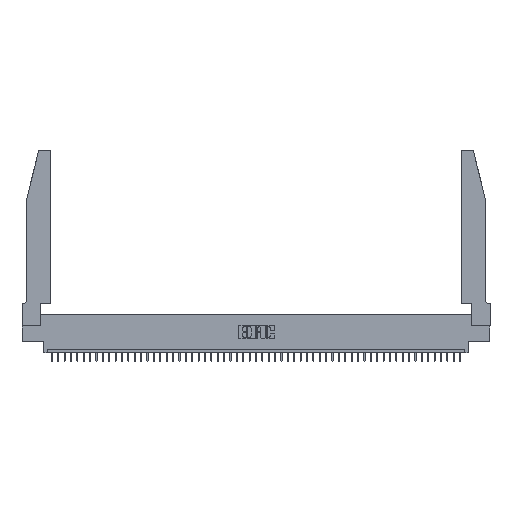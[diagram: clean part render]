
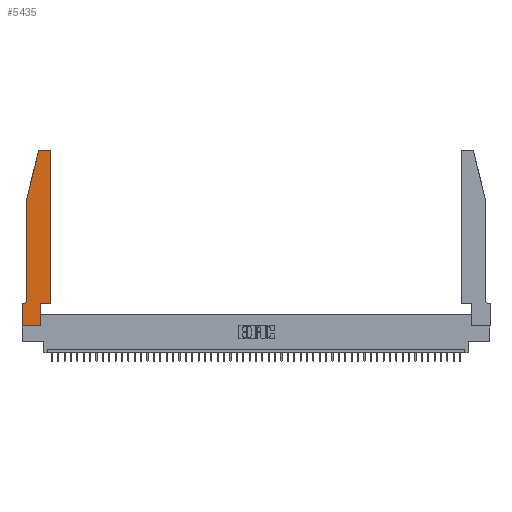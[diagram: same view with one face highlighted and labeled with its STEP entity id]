
A CAD part, top view. The second image highlights one B-rep face of the part: STEP entity #5435.
In plain terms, the highlighted planar face has unit normal (0, 0, 1).
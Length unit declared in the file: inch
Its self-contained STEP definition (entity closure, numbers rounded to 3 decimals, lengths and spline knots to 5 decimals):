
#126 = EDGE_CURVE ( 'NONE', #18314, #700, #9618, .T. ) ;
#479 = LINE ( 'NONE', #7968, #13682 ) ;
#640 = AXIS2_PLACEMENT_3D ( 'NONE', #26061, #41718, #37864 ) ;
#659 = LINE ( 'NONE', #17778, #2431 ) ;
#700 = VERTEX_POINT ( 'NONE', #10744 ) ;
#763 = EDGE_LOOP ( 'NONE', ( #3372, #18200, #48380, #49250, #43795, #35505, #13718, #44200, #23220, #9149, #31570, #44860 ) ) ;
#1346 = DIRECTION ( 'NONE',  ( -1., 0., 0. ) ) ;
#1388 = CARTESIAN_POINT ( 'NONE',  ( 0.284, 2.75, 0.37 ) ) ;
#1548 = LINE ( 'NONE', #32106, #7323 ) ;
#1636 = LINE ( 'NONE', #20898, #10021 ) ;
#2431 = VECTOR ( 'NONE', #41134, 39.37008 ) ;
#3085 = CARTESIAN_POINT ( 'NONE',  ( 0.284, 2.72, 0.37 ) ) ;
#3107 = EDGE_CURVE ( 'NONE', #9835, #30262, #40892, .T. ) ;
#3169 = CARTESIAN_POINT ( 'NONE',  ( 0., 0., 0.37 ) ) ;
#3372 = ORIENTED_EDGE ( 'NONE', *, *, #34492, .T. ) ;
#5435 = ADVANCED_FACE ( 'NONE', ( #43618 ), #12787, .T. ) ;
#5452 = LINE ( 'NONE', #35508, #43209 ) ;
#6507 = AXIS2_PLACEMENT_3D ( 'NONE', #3085, #26442, #22083 ) ;
#7140 = CIRCLE ( 'NONE', #43243, 0.07 ) ;
#7323 = VECTOR ( 'NONE', #8984, 39.37008 ) ;
#7968 = CARTESIAN_POINT ( 'NONE',  ( 0.2865, 0.35, 0.37 ) ) ;
#8028 = EDGE_CURVE ( 'NONE', #30262, #34007, #7140, .T. ) ;
#8446 = DIRECTION ( 'NONE',  ( 0., 1., 0. ) ) ;
#8984 = DIRECTION ( 'NONE',  ( 1., 0., 0. ) ) ;
#9149 = ORIENTED_EDGE ( 'NONE', *, *, #29327, .T. ) ;
#9618 = LINE ( 'NONE', #44075, #29202 ) ;
#9796 = CARTESIAN_POINT ( 'NONE',  ( 0.0755, 2., 0.37 ) ) ;
#9835 = VERTEX_POINT ( 'NONE', #41067 ) ;
#10021 = VECTOR ( 'NONE', #12682, 39.37008 ) ;
#10744 = CARTESIAN_POINT ( 'NONE',  ( 0.4505, 2.72, 0.37 ) ) ;
#11304 = CIRCLE ( 'NONE', #640, 0.03 ) ;
#11885 = LINE ( 'NONE', #36022, #16655 ) ;
#12513 = EDGE_CURVE ( 'NONE', #42675, #17325, #28645, .T. ) ;
#12682 = DIRECTION ( 'NONE',  ( 0., -1., 0. ) ) ;
#12787 = PLANE ( 'NONE',  #32257 ) ;
#12804 = DIRECTION ( 'NONE',  ( -1., 0., 0. ) ) ;
#13682 = VECTOR ( 'NONE', #8446, 39.37008 ) ;
#13718 = ORIENTED_EDGE ( 'NONE', *, *, #16114, .T. ) ;
#16114 = EDGE_CURVE ( 'NONE', #30163, #46827, #1636, .T. ) ;
#16655 = VECTOR ( 'NONE', #32419, 39.37008 ) ;
#17325 = VERTEX_POINT ( 'NONE', #37771 ) ;
#17329 = CARTESIAN_POINT ( 'NONE',  ( 0.2865, 0., 0.37 ) ) ;
#17778 = CARTESIAN_POINT ( 'NONE',  ( 0.0755, 2., 0.37 ) ) ;
#18200 = ORIENTED_EDGE ( 'NONE', *, *, #12513, .T. ) ;
#18314 = VERTEX_POINT ( 'NONE', #38909 ) ;
#18404 = VERTEX_POINT ( 'NONE', #27114 ) ;
#20594 = EDGE_CURVE ( 'NONE', #33729, #27259, #479, .T. ) ;
#20898 = CARTESIAN_POINT ( 'NONE',  ( 0., 0., 0.37 ) ) ;
#21262 = DIRECTION ( 'NONE',  ( 1., 0., 0. ) ) ;
#22083 = DIRECTION ( 'NONE',  ( 1., 0., 0. ) ) ;
#23220 = ORIENTED_EDGE ( 'NONE', *, *, #20594, .T. ) ;
#23420 = VECTOR ( 'NONE', #36781, 39.37008 ) ;
#23658 = DIRECTION ( 'NONE',  ( -1., 0., 0. ) ) ;
#24101 = DIRECTION ( 'NONE',  ( 0., 0., 1. ) ) ;
#25031 = EDGE_CURVE ( 'NONE', #46827, #33729, #1548, .T. ) ;
#25378 = CARTESIAN_POINT ( 'NONE',  ( 0.0055, 0.42, 0.37 ) ) ;
#25782 = EDGE_CURVE ( 'NONE', #17325, #9835, #659, .T. ) ;
#26061 = CARTESIAN_POINT ( 'NONE',  ( 0.4205, 2.72, 0.37 ) ) ;
#26442 = DIRECTION ( 'NONE',  ( 0., 0., 1. ) ) ;
#27114 = CARTESIAN_POINT ( 'NONE',  ( 0.4205, 2.75, 0.37 ) ) ;
#27259 = VERTEX_POINT ( 'NONE', #29152 ) ;
#27809 = CARTESIAN_POINT ( 'NONE',  ( 0.0055, 0.35, 0.37 ) ) ;
#28452 = CARTESIAN_POINT ( 'NONE',  ( 0., 0.35, 0.37 ) ) ;
#28645 = CIRCLE ( 'NONE', #6507, 0.03 ) ;
#29152 = CARTESIAN_POINT ( 'NONE',  ( 0.2865, 0.35, 0.37 ) ) ;
#29202 = VECTOR ( 'NONE', #43819, 39.37008 ) ;
#29327 = EDGE_CURVE ( 'NONE', #27259, #18314, #11885, .T. ) ;
#30163 = VERTEX_POINT ( 'NONE', #42110 ) ;
#30262 = VERTEX_POINT ( 'NONE', #35903 ) ;
#30346 = LINE ( 'NONE', #48251, #43288 ) ;
#31570 = ORIENTED_EDGE ( 'NONE', *, *, #126, .T. ) ;
#32106 = CARTESIAN_POINT ( 'NONE',  ( 0., 0., 0.37 ) ) ;
#32257 = AXIS2_PLACEMENT_3D ( 'NONE', #28452, #24101, #21262 ) ;
#32419 = DIRECTION ( 'NONE',  ( 1., 0., 0. ) ) ;
#33323 = DIRECTION ( 'NONE',  ( 0., 0., -1. ) ) ;
#33729 = VERTEX_POINT ( 'NONE', #17329 ) ;
#34007 = VERTEX_POINT ( 'NONE', #27809 ) ;
#34074 = EDGE_CURVE ( 'NONE', #34007, #30163, #5452, .T. ) ;
#34492 = EDGE_CURVE ( 'NONE', #18404, #42675, #30346, .T. ) ;
#35203 = EDGE_CURVE ( 'NONE', #700, #18404, #11304, .T. ) ;
#35505 = ORIENTED_EDGE ( 'NONE', *, *, #34074, .T. ) ;
#35508 = CARTESIAN_POINT ( 'NONE',  ( 0.0755, 0.35, 0.37 ) ) ;
#35903 = CARTESIAN_POINT ( 'NONE',  ( 0.0755, 0.42, 0.37 ) ) ;
#36022 = CARTESIAN_POINT ( 'NONE',  ( 0.4505, 0.35, 0.37 ) ) ;
#36781 = DIRECTION ( 'NONE',  ( 0., -1., 0. ) ) ;
#37771 = CARTESIAN_POINT ( 'NONE',  ( 0.25487, 2.72718, 0.37 ) ) ;
#37864 = DIRECTION ( 'NONE',  ( 1., 0., 0. ) ) ;
#38909 = CARTESIAN_POINT ( 'NONE',  ( 0.4505, 0.35, 0.37 ) ) ;
#40892 = LINE ( 'NONE', #9796, #23420 ) ;
#41067 = CARTESIAN_POINT ( 'NONE',  ( 0.0755, 2., 0.37 ) ) ;
#41134 = DIRECTION ( 'NONE',  ( -0.239, -0.971, 0. ) ) ;
#41718 = DIRECTION ( 'NONE',  ( 0., 0., 1. ) ) ;
#42110 = CARTESIAN_POINT ( 'NONE',  ( 0., 0.35, 0.37 ) ) ;
#42675 = VERTEX_POINT ( 'NONE', #1388 ) ;
#43209 = VECTOR ( 'NONE', #1346, 39.37008 ) ;
#43243 = AXIS2_PLACEMENT_3D ( 'NONE', #25378, #33323, #12804 ) ;
#43288 = VECTOR ( 'NONE', #23658, 39.37008 ) ;
#43618 = FACE_OUTER_BOUND ( 'NONE', #763, .T. ) ;
#43795 = ORIENTED_EDGE ( 'NONE', *, *, #8028, .T. ) ;
#43819 = DIRECTION ( 'NONE',  ( 0., 1., 0. ) ) ;
#44075 = CARTESIAN_POINT ( 'NONE',  ( 0.4505, 0.35, 0.37 ) ) ;
#44200 = ORIENTED_EDGE ( 'NONE', *, *, #25031, .T. ) ;
#44860 = ORIENTED_EDGE ( 'NONE', *, *, #35203, .T. ) ;
#46827 = VERTEX_POINT ( 'NONE', #3169 ) ;
#48251 = CARTESIAN_POINT ( 'NONE',  ( 0.2605, 2.75, 0.37 ) ) ;
#48380 = ORIENTED_EDGE ( 'NONE', *, *, #25782, .T. ) ;
#49250 = ORIENTED_EDGE ( 'NONE', *, *, #3107, .T. ) ;
